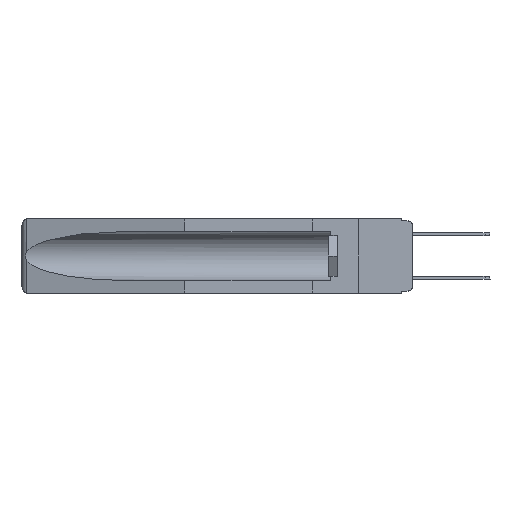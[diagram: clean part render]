
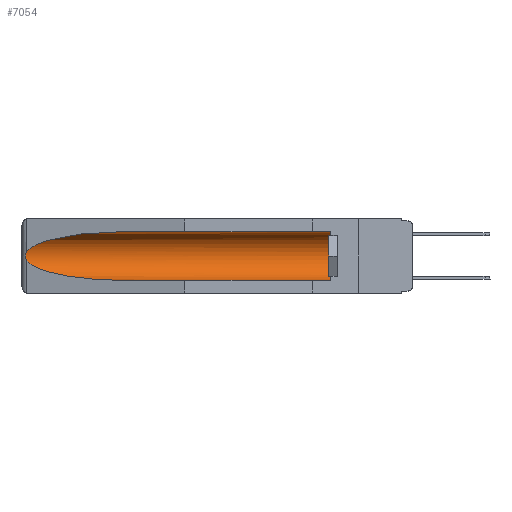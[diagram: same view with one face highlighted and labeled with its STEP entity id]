
A CAD part, left-side view. The second image highlights one B-rep face of the part: STEP entity #7054.
In plain terms, the highlighted cylindrical face has radius 2.857 mm (diameter 5.715 mm), a partial arc.
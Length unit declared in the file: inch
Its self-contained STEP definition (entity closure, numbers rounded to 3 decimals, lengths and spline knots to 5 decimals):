
#371 = ORIENTED_EDGE ( 'NONE', *, *, #13730, .T. ) ;
#1034 = CARTESIAN_POINT ( 'NONE',  ( 0.155, 1.07973, -0.059 ) ) ;
#1239 = CARTESIAN_POINT ( 'NONE',  ( 0.26597, 1.52961, -0.15275 ) ) ;
#1967 = VERTEX_POINT ( 'NONE', #13360 ) ;
#2660 = EDGE_CURVE ( 'NONE', #1967, #4202, #6817, .T. ) ;
#3464 = CARTESIAN_POINT ( 'NONE',  ( 0.21114, 1.30732, -0.284 ) ) ;
#3649 = EDGE_LOOP ( 'NONE', ( #371, #27698, #8715, #26964, #8959, #12867 ) ) ;
#4202 = VERTEX_POINT ( 'NONE', #18174 ) ;
#5560 = CARTESIAN_POINT ( 'NONE',  ( 0.2675, 1.53308, -0.16763 ) ) ;
#6817 = CIRCLE ( 'NONE', #11390, 0.1125 ) ;
#7054 = ADVANCED_FACE ( 'NONE', ( #18706 ), #27444, .F. ) ;
#7080 = EDGE_CURVE ( 'NONE', #1967, #22762, #28274, .T. ) ;
#7196 = CARTESIAN_POINT ( 'NONE',  ( 0.26537, 1.52718, -0.19328 ) ) ;
#7390 = LINE ( 'NONE', #18367, #23022 ) ;
#7730 = CARTESIAN_POINT ( 'NONE',  ( 0.26537, 1.52718, -0.14972 ) ) ;
#7892 = CARTESIAN_POINT ( 'NONE',  ( 0.155, -0.30754, -0.1715 ) ) ;
#8494 = CARTESIAN_POINT ( 'NONE',  ( 0.155, 1.07973, -0.284 ) ) ;
#8539 = CARTESIAN_POINT ( 'NONE',  ( 0.155, 1.07973, -0.059 ) ) ;
#8715 = ORIENTED_EDGE ( 'NONE', *, *, #12767, .T. ) ;
#8959 = ORIENTED_EDGE ( 'NONE', *, *, #2660, .T. ) ;
#9004 = EDGE_CURVE ( 'NONE', #4202, #24741, #7390, .T. ) ;
#9495 = CARTESIAN_POINT ( 'NONE',  ( 0.155, 1.07973, -0.284 ) ) ;
#11390 = AXIS2_PLACEMENT_3D ( 'NONE', #15450, #17847, #19999 ) ;
#11942 = CARTESIAN_POINT ( 'NONE',  ( 0.25451, 1.48313, -0.09465 ) ) ;
#12283 = CARTESIAN_POINT ( 'NONE',  ( 0.2673, 1.53269, -0.17917 ) ) ;
#12767 = EDGE_CURVE ( 'NONE', #14316, #22762, #14495, .T. ) ;
#12867 = ORIENTED_EDGE ( 'NONE', *, *, #9004, .T. ) ;
#13360 = CARTESIAN_POINT ( 'NONE',  ( 0.155, 0.126, -0.284 ) ) ;
#13613 = CARTESIAN_POINT ( 'NONE',  ( 0.26537, 1.52718, -0.14972 ) ) ;
#13730 = EDGE_CURVE ( 'NONE', #24741, #15281, #27415, .T. ) ;
#13795 = AXIS2_PLACEMENT_3D ( 'NONE', #7892, #16584, #14458 ) ;
#14103 = CARTESIAN_POINT ( 'NONE',  ( 0.26537, 1.52718, -0.14972 ) ) ;
#14301 = CARTESIAN_POINT ( 'NONE',  ( 0.26597, 1.5296, -0.19026 ) ) ;
#14316 = VERTEX_POINT ( 'NONE', #20623 ) ;
#14458 = DIRECTION ( 'NONE',  ( 0., 0., 1. ) ) ;
#14495 =( BOUNDED_CURVE ( )  B_SPLINE_CURVE ( 3, ( #7196, #22766, #3464, #9495 ),
 .UNSPECIFIED., .F., .F. ) 
 B_SPLINE_CURVE_WITH_KNOTS ( ( 4, 4 ),
 ( 0.1948, 1.5708 ),
 .UNSPECIFIED. ) 
 CURVE ( )  GEOMETRIC_REPRESENTATION_ITEM ( )  RATIONAL_B_SPLINE_CURVE ( ( 1., 0.848, 0.848, 1. ) ) 
 REPRESENTATION_ITEM ( '' )  );
#15281 = VERTEX_POINT ( 'NONE', #13613 ) ;
#15450 = CARTESIAN_POINT ( 'NONE',  ( 0.155, 0.126, -0.1715 ) ) ;
#15957 = DIRECTION ( 'NONE',  ( 0., 1., 0. ) ) ;
#16584 = DIRECTION ( 'NONE',  ( 0., 1., 0. ) ) ;
#16977 = VECTOR ( 'NONE', #26273, 39.37008 ) ;
#17261 = CARTESIAN_POINT ( 'NONE',  ( 0.155, -0.30754, -0.284 ) ) ;
#17847 = DIRECTION ( 'NONE',  ( 0., -1., 0. ) ) ;
#18174 = CARTESIAN_POINT ( 'NONE',  ( 0.155, 0.126, -0.059 ) ) ;
#18367 = CARTESIAN_POINT ( 'NONE',  ( 0.155, -0.30754, -0.059 ) ) ;
#18416 = CARTESIAN_POINT ( 'NONE',  ( 0.2673, 1.5327, -0.16383 ) ) ;
#18564 = CARTESIAN_POINT ( 'NONE',  ( 0.26655, 1.53094, -0.18657 ) ) ;
#18706 = FACE_OUTER_BOUND ( 'NONE', #3649, .T. ) ;
#19999 = DIRECTION ( 'NONE',  ( 0., 0., 1. ) ) ;
#20623 = CARTESIAN_POINT ( 'NONE',  ( 0.26537, 1.52718, -0.19328 ) ) ;
#20721 = CARTESIAN_POINT ( 'NONE',  ( 0.26654, 1.53092, -0.15636 ) ) ;
#22762 = VERTEX_POINT ( 'NONE', #8494 ) ;
#22766 = CARTESIAN_POINT ( 'NONE',  ( 0.25451, 1.48313, -0.24835 ) ) ;
#22807 = CARTESIAN_POINT ( 'NONE',  ( 0.21114, 1.30732, -0.059 ) ) ;
#22858 = CARTESIAN_POINT ( 'NONE',  ( 0.2675, 1.53308, -0.17534 ) ) ;
#23022 = VECTOR ( 'NONE', #15957, 39.37008 ) ;
#23442 = EDGE_CURVE ( 'NONE', #15281, #14316, #24002, .T. ) ;
#24002 = B_SPLINE_CURVE_WITH_KNOTS ( 'NONE', 3,
 ( #7730, #1239, #20721, #18416, #5560, #22858, #12283, #18564, #14301, #27148 ),
 .UNSPECIFIED., .F., .F.,
 ( 4, 2, 2, 2, 4 ),
 ( 0., 0.00029, 0.00058, 0.00087, 0.00117 ),
 .UNSPECIFIED. ) ;
#24741 = VERTEX_POINT ( 'NONE', #8539 ) ;
#26273 = DIRECTION ( 'NONE',  ( 0., 1., 0. ) ) ;
#26964 = ORIENTED_EDGE ( 'NONE', *, *, #7080, .F. ) ;
#27148 = CARTESIAN_POINT ( 'NONE',  ( 0.26537, 1.52718, -0.19328 ) ) ;
#27415 =( BOUNDED_CURVE ( )  B_SPLINE_CURVE ( 3, ( #1034, #22807, #11942, #14103 ),
 .UNSPECIFIED., .F., .F. ) 
 B_SPLINE_CURVE_WITH_KNOTS ( ( 4, 4 ),
 ( 4.71239, 6.08839 ),
 .UNSPECIFIED. ) 
 CURVE ( )  GEOMETRIC_REPRESENTATION_ITEM ( )  RATIONAL_B_SPLINE_CURVE ( ( 1., 0.848, 0.848, 1. ) ) 
 REPRESENTATION_ITEM ( '' )  );
#27444 = CYLINDRICAL_SURFACE ( 'NONE', #13795, 0.1125 ) ;
#27698 = ORIENTED_EDGE ( 'NONE', *, *, #23442, .T. ) ;
#28274 = LINE ( 'NONE', #17261, #16977 ) ;
